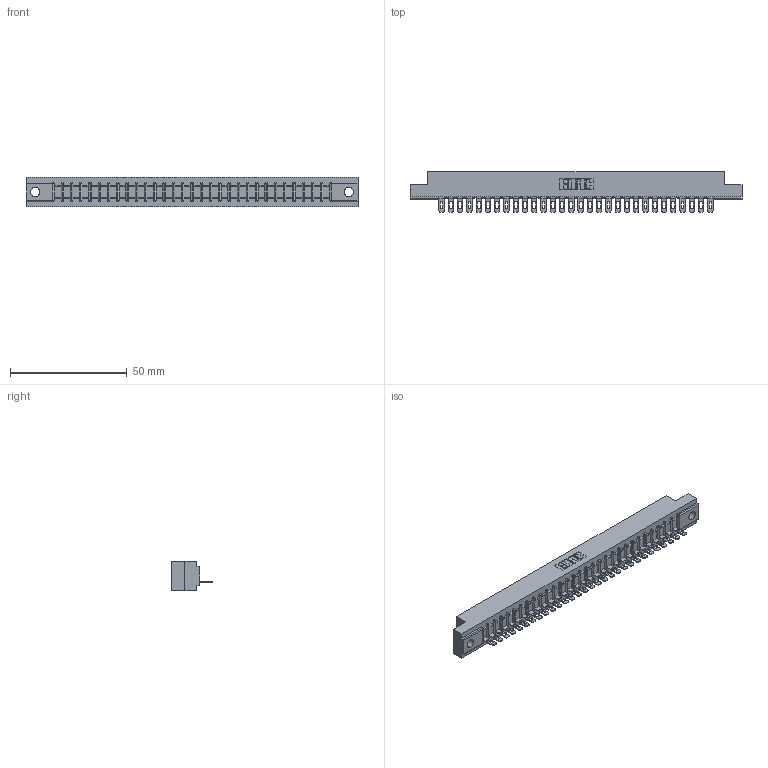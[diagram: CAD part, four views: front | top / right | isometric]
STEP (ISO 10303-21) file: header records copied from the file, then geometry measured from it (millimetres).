
FILE_DESCRIPTION (( 'STEP AP203' ), '1' );
FILE_NAME ('307-030-501-104.STEP', '2019-09-05T04:01:11', ( '' ), ( '' ), 'SwSTEP 2.0', 'SolidWorks 2016', '' );
FILE_SCHEMA (( 'CONFIG_CONTROL_DESIGN' ));
Length unit declared in the file: inch
Products named in the file (3): 307-290-002_501; 307-030-501-104; 307 Part_.156 Dia Mounting Holes
Assembly tree (31 placements, depth 2):
  307-030-501-104
    307 Part_.156 Dia Mounting Holes
    307-290-002_501  x30
Bounding box: 141.88 x 17.42 x 12.7 mm (x, y, z)
Volume: 15014.1 mm3; surface area: 18653.9 mm2
Topology: 31 solids, 31 shells, 2443 faces, 7499 edges, 4914 vertices
Faces by surface type: plane 1404, cylinder 977, sphere 62
Entity records: 28410 total; most frequent: CARTESIAN_POINT 4794, ORIENTED_EDGE 4782, DIRECTION 4659, EDGE_CURVE 2391, VECTOR 1829, LINE 1829, VERTEX_POINT 1550, AXIS2_PLACEMENT_3D 1415
